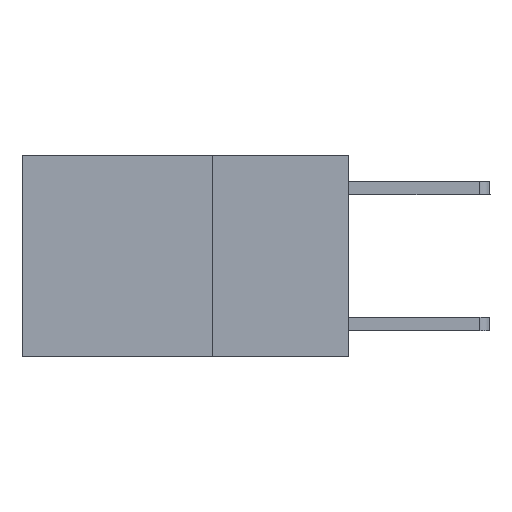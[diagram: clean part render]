
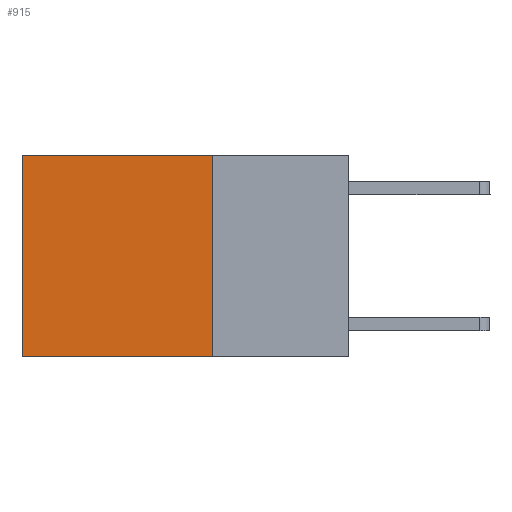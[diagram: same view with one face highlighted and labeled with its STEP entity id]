
A CAD part, left-side view. The second image highlights one B-rep face of the part: STEP entity #915.
In plain terms, the highlighted planar face has unit normal (-1, 0, 0).
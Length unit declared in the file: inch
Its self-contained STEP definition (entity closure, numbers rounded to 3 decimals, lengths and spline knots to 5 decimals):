
#785 = EDGE_LOOP ( 'NONE', ( #9043, #6890, #9317, #3038 ) ) ;
#915 = ADVANCED_FACE ( 'NONE', ( #6047 ), #11089, .F. ) ;
#1217 = DIRECTION ( 'NONE',  ( 0., 1., 0. ) ) ;
#2516 = EDGE_CURVE ( 'NONE', #7909, #9358, #3834, .T. ) ;
#2520 = LINE ( 'NONE', #6852, #5036 ) ;
#3038 = ORIENTED_EDGE ( 'NONE', *, *, #9343, .T. ) ;
#3403 = EDGE_CURVE ( 'NONE', #3710, #9358, #4416, .T. ) ;
#3710 = VERTEX_POINT ( 'NONE', #11884 ) ;
#3834 = LINE ( 'NONE', #4114, #6028 ) ;
#4114 = CARTESIAN_POINT ( 'NONE',  ( 0.2625, 0.6, 0. ) ) ;
#4416 = LINE ( 'NONE', #7942, #6923 ) ;
#4678 = CARTESIAN_POINT ( 'NONE',  ( 0.2625, 0.6, 0. ) ) ;
#4713 = CARTESIAN_POINT ( 'NONE',  ( 0.2625, 0.25, 0. ) ) ;
#4928 = VECTOR ( 'NONE', #6191, 39.37008 ) ;
#5036 = VECTOR ( 'NONE', #7774, 39.37008 ) ;
#5642 = DIRECTION ( 'NONE',  ( 0., 0., -1. ) ) ;
#6028 = VECTOR ( 'NONE', #8432, 39.37008 ) ;
#6047 = FACE_OUTER_BOUND ( 'NONE', #785, .T. ) ;
#6191 = DIRECTION ( 'NONE',  ( 0., 0., -1. ) ) ;
#6852 = CARTESIAN_POINT ( 'NONE',  ( 0.2625, 0.25, 0. ) ) ;
#6890 = ORIENTED_EDGE ( 'NONE', *, *, #3403, .F. ) ;
#6901 = CARTESIAN_POINT ( 'NONE',  ( 0.2625, 0.6, -0.37 ) ) ;
#6923 = VECTOR ( 'NONE', #1217, 39.37008 ) ;
#7623 = EDGE_CURVE ( 'NONE', #8214, #3710, #7731, .T. ) ;
#7731 = LINE ( 'NONE', #9860, #4928 ) ;
#7774 = DIRECTION ( 'NONE',  ( 0., 1., 0. ) ) ;
#7909 = VERTEX_POINT ( 'NONE', #4678 ) ;
#7942 = CARTESIAN_POINT ( 'NONE',  ( 0.2625, 0.25, -0.37 ) ) ;
#8214 = VERTEX_POINT ( 'NONE', #8887 ) ;
#8401 = AXIS2_PLACEMENT_3D ( 'NONE', #4713, #11128, #5642 ) ;
#8432 = DIRECTION ( 'NONE',  ( 0., 0., -1. ) ) ;
#8887 = CARTESIAN_POINT ( 'NONE',  ( 0.2625, 0.25, 0. ) ) ;
#9043 = ORIENTED_EDGE ( 'NONE', *, *, #2516, .T. ) ;
#9317 = ORIENTED_EDGE ( 'NONE', *, *, #7623, .F. ) ;
#9343 = EDGE_CURVE ( 'NONE', #8214, #7909, #2520, .T. ) ;
#9358 = VERTEX_POINT ( 'NONE', #6901 ) ;
#9860 = CARTESIAN_POINT ( 'NONE',  ( 0.2625, 0.25, 0. ) ) ;
#11089 = PLANE ( 'NONE',  #8401 ) ;
#11128 = DIRECTION ( 'NONE',  ( 1., 0., 0. ) ) ;
#11884 = CARTESIAN_POINT ( 'NONE',  ( 0.2625, 0.25, -0.37 ) ) ;
